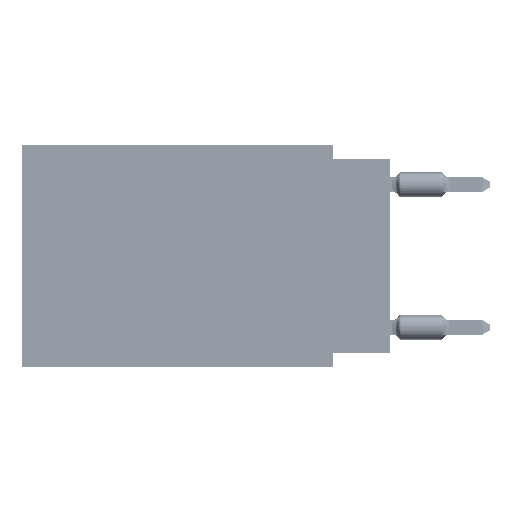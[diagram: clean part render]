
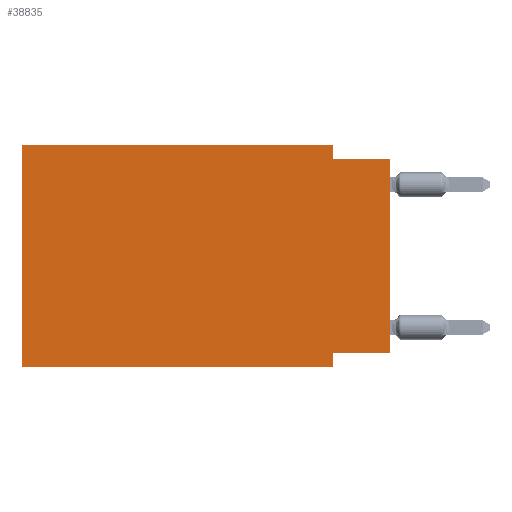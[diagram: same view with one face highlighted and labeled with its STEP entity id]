
A CAD part, left-side view. The second image highlights one B-rep face of the part: STEP entity #38835.
In plain terms, the highlighted planar face has unit normal (-1, 0, 0).
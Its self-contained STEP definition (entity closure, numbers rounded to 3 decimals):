
#4034 = CARTESIAN_POINT ( 'NONE',  ( 0., 2.54, -9.906 ) ) ;
#5123 = DIRECTION ( 'NONE',  ( 0., 1., 0. ) ) ;
#5247 = CARTESIAN_POINT ( 'NONE',  ( 0., 16.383, 0. ) ) ;
#6481 = DIRECTION ( 'NONE',  ( 0., -1., 0. ) ) ;
#6987 = CARTESIAN_POINT ( 'NONE',  ( 0., 2.54, 0. ) ) ;
#7996 = EDGE_CURVE ( 'NONE', #57103, #58638, #23792, .T. ) ;
#9107 = ORIENTED_EDGE ( 'NONE', *, *, #66009, .T. ) ;
#9637 = DIRECTION ( 'NONE',  ( 0., 0., 1. ) ) ;
#10852 = CARTESIAN_POINT ( 'NONE',  ( 0., 2.54, -9.271 ) ) ;
#11966 = VECTOR ( 'NONE', #69922, 1000. ) ;
#12403 = LINE ( 'NONE', #5247, #72705 ) ;
#15661 = VECTOR ( 'NONE', #5123, 1000. ) ;
#17896 = DIRECTION ( 'NONE',  ( 0., 0., 1. ) ) ;
#18270 = VERTEX_POINT ( 'NONE', #34094 ) ;
#18542 = LINE ( 'NONE', #44207, #11966 ) ;
#22674 = LINE ( 'NONE', #79968, #26381 ) ;
#23792 = LINE ( 'NONE', #49463, #60422 ) ;
#25934 = DIRECTION ( 'NONE',  ( 0., 0., -1. ) ) ;
#26381 = VECTOR ( 'NONE', #9637, 1000. ) ;
#30936 = VERTEX_POINT ( 'NONE', #37935 ) ;
#32373 = EDGE_LOOP ( 'NONE', ( #9107, #40830, #76654, #57849, #75122, #69269, #61053, #57383 ) ) ;
#32991 = EDGE_CURVE ( 'NONE', #18270, #57103, #12403, .T. ) ;
#33005 = DIRECTION ( 'NONE',  ( 0., 0., -1. ) ) ;
#34094 = CARTESIAN_POINT ( 'NONE',  ( 0., 16.383, -9.906 ) ) ;
#35024 = DIRECTION ( 'NONE',  ( 0., 0., -1. ) ) ;
#37935 = CARTESIAN_POINT ( 'NONE',  ( 0., 0., -9.271 ) ) ;
#38835 = ADVANCED_FACE ( 'NONE', ( #50284 ), #43978, .F. ) ;
#40830 = ORIENTED_EDGE ( 'NONE', *, *, #62015, .F. ) ;
#43147 = VERTEX_POINT ( 'NONE', #4034 ) ;
#43978 = PLANE ( 'NONE',  #81461 ) ;
#44207 = CARTESIAN_POINT ( 'NONE',  ( 0., 16.383, -9.906 ) ) ;
#46869 = LINE ( 'NONE', #59527, #76939 ) ;
#48413 = EDGE_CURVE ( 'NONE', #78783, #43147, #81313, .T. ) ;
#48472 = CARTESIAN_POINT ( 'NONE',  ( 0., 2.54, -9.906 ) ) ;
#49463 = CARTESIAN_POINT ( 'NONE',  ( 0., 16.383, 0. ) ) ;
#50284 = FACE_OUTER_BOUND ( 'NONE', #32373, .T. ) ;
#50709 = DIRECTION ( 'NONE',  ( 1., 0., 0. ) ) ;
#51116 = EDGE_CURVE ( 'NONE', #30936, #78783, #81361, .T. ) ;
#52348 = DIRECTION ( 'NONE',  ( 0., -1., 0. ) ) ;
#54115 = EDGE_CURVE ( 'NONE', #18270, #43147, #18542, .T. ) ;
#55615 = CARTESIAN_POINT ( 'NONE',  ( 0., 0., -0.635 ) ) ;
#56083 = CARTESIAN_POINT ( 'NONE',  ( 0., 0., -9.271 ) ) ;
#57103 = VERTEX_POINT ( 'NONE', #74986 ) ;
#57383 = ORIENTED_EDGE ( 'NONE', *, *, #51116, .F. ) ;
#57849 = ORIENTED_EDGE ( 'NONE', *, *, #7996, .F. ) ;
#58638 = VERTEX_POINT ( 'NONE', #66529 ) ;
#59009 = VERTEX_POINT ( 'NONE', #72671 ) ;
#59527 = CARTESIAN_POINT ( 'NONE',  ( 0., 0., -0.635 ) ) ;
#60422 = VECTOR ( 'NONE', #6481, 1000. ) ;
#60955 = VECTOR ( 'NONE', #25934, 1000. ) ;
#61053 = ORIENTED_EDGE ( 'NONE', *, *, #48413, .F. ) ;
#61431 = EDGE_CURVE ( 'NONE', #58638, #59009, #71015, .T. ) ;
#62015 = EDGE_CURVE ( 'NONE', #59009, #73936, #46869, .T. ) ;
#65052 = VECTOR ( 'NONE', #35024, 1000. ) ;
#66009 = EDGE_CURVE ( 'NONE', #30936, #73936, #22674, .T. ) ;
#66529 = CARTESIAN_POINT ( 'NONE',  ( 0., 2.54, 0. ) ) ;
#69269 = ORIENTED_EDGE ( 'NONE', *, *, #54115, .T. ) ;
#69692 = CARTESIAN_POINT ( 'NONE',  ( 0., 16.383, 0. ) ) ;
#69922 = DIRECTION ( 'NONE',  ( 0., -1., 0. ) ) ;
#71015 = LINE ( 'NONE', #6987, #60955 ) ;
#72671 = CARTESIAN_POINT ( 'NONE',  ( 0., 2.54, -0.635 ) ) ;
#72705 = VECTOR ( 'NONE', #17896, 1000. ) ;
#73936 = VERTEX_POINT ( 'NONE', #55615 ) ;
#74986 = CARTESIAN_POINT ( 'NONE',  ( 0., 16.383, 0. ) ) ;
#75122 = ORIENTED_EDGE ( 'NONE', *, *, #32991, .F. ) ;
#76654 = ORIENTED_EDGE ( 'NONE', *, *, #61431, .F. ) ;
#76939 = VECTOR ( 'NONE', #52348, 1000. ) ;
#78783 = VERTEX_POINT ( 'NONE', #10852 ) ;
#79968 = CARTESIAN_POINT ( 'NONE',  ( 0., 0., 0. ) ) ;
#81313 = LINE ( 'NONE', #48472, #65052 ) ;
#81361 = LINE ( 'NONE', #56083, #15661 ) ;
#81461 = AXIS2_PLACEMENT_3D ( 'NONE', #69692, #50709, #33005 ) ;
